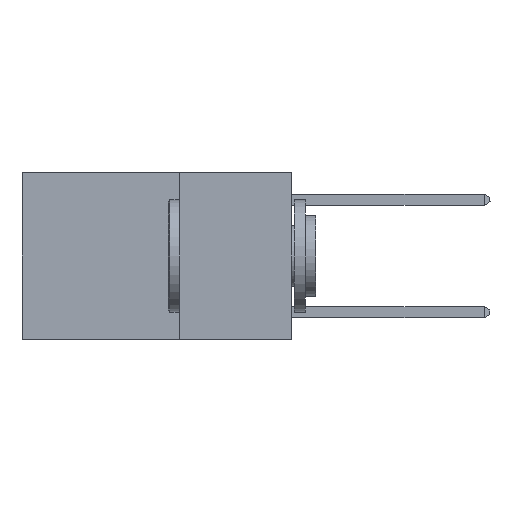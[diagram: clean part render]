
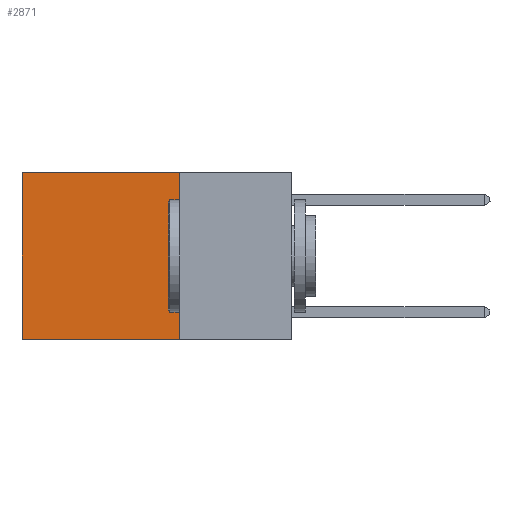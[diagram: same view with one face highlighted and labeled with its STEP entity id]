
A CAD part, left-side view. The second image highlights one B-rep face of the part: STEP entity #2871.
In plain terms, the highlighted planar face has unit normal (-1, 0, 0).
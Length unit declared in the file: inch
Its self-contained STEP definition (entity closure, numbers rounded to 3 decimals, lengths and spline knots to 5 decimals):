
#66 = CARTESIAN_POINT ( 'NONE',  ( 0.2625, 0.25, 0. ) ) ;
#501 = VECTOR ( 'NONE', #5247, 39.37008 ) ;
#1287 = AXIS2_PLACEMENT_3D ( 'NONE', #2068, #2816, #8192 ) ;
#1592 = EDGE_CURVE ( 'NONE', #5531, #7761, #4243, .T. ) ;
#1866 = LINE ( 'NONE', #66, #7544 ) ;
#2053 = VECTOR ( 'NONE', #3063, 39.37008 ) ;
#2068 = CARTESIAN_POINT ( 'NONE',  ( 0.2625, 0.25, 0. ) ) ;
#2323 = EDGE_CURVE ( 'NONE', #7719, #7761, #2751, .T. ) ;
#2395 = EDGE_CURVE ( 'NONE', #9403, #5531, #5969, .T. ) ;
#2751 = LINE ( 'NONE', #6008, #501 ) ;
#2816 = DIRECTION ( 'NONE',  ( 1., 0., 0. ) ) ;
#2871 = ADVANCED_FACE ( 'NONE', ( #7479 ), #8885, .F. ) ;
#3063 = DIRECTION ( 'NONE',  ( 0., 0., -1. ) ) ;
#3147 = ORIENTED_EDGE ( 'NONE', *, *, #1592, .F. ) ;
#3282 = CARTESIAN_POINT ( 'NONE',  ( 0.2625, 0.25, -0.37 ) ) ;
#4243 = LINE ( 'NONE', #7133, #8245 ) ;
#4258 = ORIENTED_EDGE ( 'NONE', *, *, #2395, .F. ) ;
#4512 = ORIENTED_EDGE ( 'NONE', *, *, #9763, .T. ) ;
#4774 = ORIENTED_EDGE ( 'NONE', *, *, #2323, .T. ) ;
#5153 = CARTESIAN_POINT ( 'NONE',  ( 0.2625, 0.25, 0. ) ) ;
#5247 = DIRECTION ( 'NONE',  ( 0., 0., -1. ) ) ;
#5531 = VERTEX_POINT ( 'NONE', #3282 ) ;
#5969 = LINE ( 'NONE', #7696, #2053 ) ;
#6008 = CARTESIAN_POINT ( 'NONE',  ( 0.2625, 0.6, 0. ) ) ;
#6283 = DIRECTION ( 'NONE',  ( 0., 1., 0. ) ) ;
#7133 = CARTESIAN_POINT ( 'NONE',  ( 0.2625, 0.25, -0.37 ) ) ;
#7437 = EDGE_LOOP ( 'NONE', ( #4774, #3147, #4258, #4512 ) ) ;
#7479 = FACE_OUTER_BOUND ( 'NONE', #7437, .T. ) ;
#7544 = VECTOR ( 'NONE', #6283, 39.37008 ) ;
#7696 = CARTESIAN_POINT ( 'NONE',  ( 0.2625, 0.25, 0. ) ) ;
#7719 = VERTEX_POINT ( 'NONE', #9588 ) ;
#7761 = VERTEX_POINT ( 'NONE', #8229 ) ;
#7975 = DIRECTION ( 'NONE',  ( 0., 1., 0. ) ) ;
#8192 = DIRECTION ( 'NONE',  ( 0., 0., -1. ) ) ;
#8229 = CARTESIAN_POINT ( 'NONE',  ( 0.2625, 0.6, -0.37 ) ) ;
#8245 = VECTOR ( 'NONE', #7975, 39.37008 ) ;
#8885 = PLANE ( 'NONE',  #1287 ) ;
#9403 = VERTEX_POINT ( 'NONE', #5153 ) ;
#9588 = CARTESIAN_POINT ( 'NONE',  ( 0.2625, 0.6, 0. ) ) ;
#9763 = EDGE_CURVE ( 'NONE', #9403, #7719, #1866, .T. ) ;
